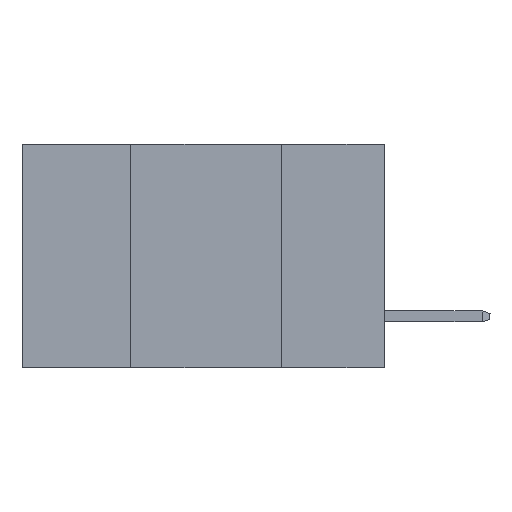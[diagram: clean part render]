
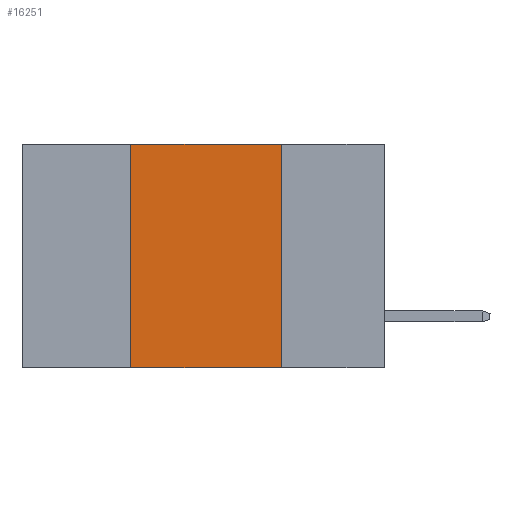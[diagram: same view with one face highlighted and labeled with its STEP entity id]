
A CAD part, left-side view. The second image highlights one B-rep face of the part: STEP entity #16251.
In plain terms, the highlighted planar face has unit normal (-1, 0, 0).
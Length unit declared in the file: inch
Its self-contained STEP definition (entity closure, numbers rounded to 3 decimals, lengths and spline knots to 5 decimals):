
#248 = PLANE ( 'NONE',  #12399 ) ;
#376 = EDGE_CURVE ( 'NONE', #4287, #10737, #7622, .T. ) ;
#445 = VECTOR ( 'NONE', #17736, 39.37008 ) ;
#706 = CARTESIAN_POINT ( 'NONE',  ( 0., 0.6, -0.37 ) ) ;
#1741 = ORIENTED_EDGE ( 'NONE', *, *, #2944, .F. ) ;
#2944 = EDGE_CURVE ( 'NONE', #18875, #10737, #3723, .T. ) ;
#3596 = ORIENTED_EDGE ( 'NONE', *, *, #376, .T. ) ;
#3723 = LINE ( 'NONE', #10697, #445 ) ;
#3740 = FACE_OUTER_BOUND ( 'NONE', #19711, .T. ) ;
#4127 = CARTESIAN_POINT ( 'NONE',  ( 0., 0.17, -0.37 ) ) ;
#4287 = VERTEX_POINT ( 'NONE', #5678 ) ;
#4659 = LINE ( 'NONE', #11649, #19116 ) ;
#5522 = CARTESIAN_POINT ( 'NONE',  ( 0., 0.17, 0. ) ) ;
#5678 = CARTESIAN_POINT ( 'NONE',  ( 0., 0.42, -0.37 ) ) ;
#5688 = CARTESIAN_POINT ( 'NONE',  ( 0., 0.6, 0. ) ) ;
#5918 = EDGE_CURVE ( 'NONE', #4287, #11584, #22117, .T. ) ;
#6375 = CARTESIAN_POINT ( 'NONE',  ( 0., 0.42, -0.37 ) ) ;
#7622 = LINE ( 'NONE', #706, #11009 ) ;
#10401 = DIRECTION ( 'NONE',  ( 0., 0., -1. ) ) ;
#10697 = CARTESIAN_POINT ( 'NONE',  ( 0., 0.17, -0.37 ) ) ;
#10737 = VERTEX_POINT ( 'NONE', #4127 ) ;
#10823 = DIRECTION ( 'NONE',  ( 1., 0., 0. ) ) ;
#11009 = VECTOR ( 'NONE', #22121, 39.37008 ) ;
#11584 = VERTEX_POINT ( 'NONE', #16366 ) ;
#11649 = CARTESIAN_POINT ( 'NONE',  ( 0., 0.6, 0. ) ) ;
#12312 = VECTOR ( 'NONE', #20381, 39.37008 ) ;
#12399 = AXIS2_PLACEMENT_3D ( 'NONE', #5688, #10823, #10401 ) ;
#16251 = ADVANCED_FACE ( 'NONE', ( #3740 ), #248, .F. ) ;
#16366 = CARTESIAN_POINT ( 'NONE',  ( 0., 0.42, 0. ) ) ;
#17605 = ORIENTED_EDGE ( 'NONE', *, *, #5918, .F. ) ;
#17736 = DIRECTION ( 'NONE',  ( 0., 0., -1. ) ) ;
#18656 = DIRECTION ( 'NONE',  ( 0., -1., 0. ) ) ;
#18875 = VERTEX_POINT ( 'NONE', #5522 ) ;
#19116 = VECTOR ( 'NONE', #18656, 39.37008 ) ;
#19711 = EDGE_LOOP ( 'NONE', ( #1741, #20176, #17605, #3596 ) ) ;
#20176 = ORIENTED_EDGE ( 'NONE', *, *, #21154, .F. ) ;
#20381 = DIRECTION ( 'NONE',  ( 0., 0., 1. ) ) ;
#21154 = EDGE_CURVE ( 'NONE', #11584, #18875, #4659, .T. ) ;
#22117 = LINE ( 'NONE', #6375, #12312 ) ;
#22121 = DIRECTION ( 'NONE',  ( 0., -1., 0. ) ) ;
